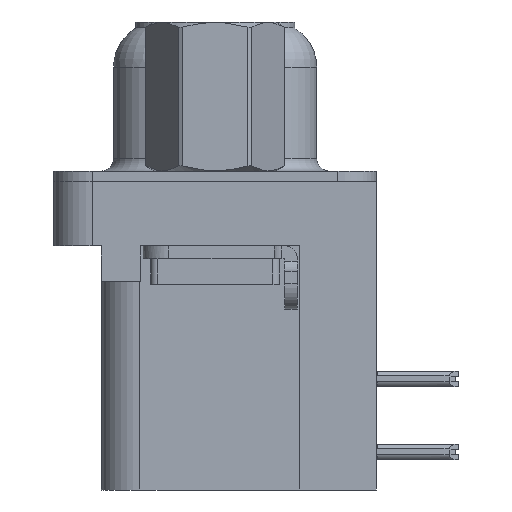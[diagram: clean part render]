
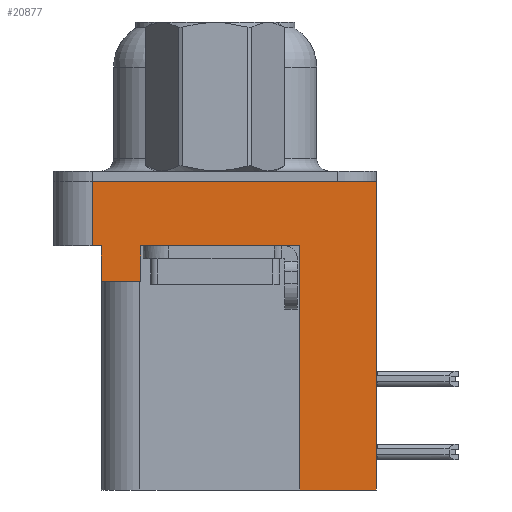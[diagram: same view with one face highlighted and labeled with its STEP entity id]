
A CAD part, left-side view. The second image highlights one B-rep face of the part: STEP entity #20877.
In plain terms, the highlighted planar face has unit normal (-1, 0, 0).
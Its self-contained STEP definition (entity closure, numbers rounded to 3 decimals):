
#188 = ORIENTED_EDGE ( 'NONE', *, *, #10107, .F. ) ;
#327 = CARTESIAN_POINT ( 'NONE',  ( -2.91, 4.425, -3.9 ) ) ;
#894 = ORIENTED_EDGE ( 'NONE', *, *, #11060, .T. ) ;
#1108 = VECTOR ( 'NONE', #5291, 1000. ) ;
#1825 = DIRECTION ( 'NONE',  ( -1., 0., 0. ) ) ;
#2499 = LINE ( 'NONE', #14747, #24921 ) ;
#2688 = VERTEX_POINT ( 'NONE', #21007 ) ;
#3097 = CARTESIAN_POINT ( 'NONE',  ( -2.91, 2.895, -3.9 ) ) ;
#3194 = CARTESIAN_POINT ( 'NONE',  ( -2.91, 4.425, -3.9 ) ) ;
#3230 = VERTEX_POINT ( 'NONE', #9483 ) ;
#3267 = EDGE_CURVE ( 'NONE', #19545, #26662, #27232, .T. ) ;
#3605 = CARTESIAN_POINT ( 'NONE',  ( -2.91, 4.775, 0. ) ) ;
#3704 = ORIENTED_EDGE ( 'NONE', *, *, #19680, .F. ) ;
#3822 = CARTESIAN_POINT ( 'NONE',  ( -2.91, 4.775, -2.5 ) ) ;
#3867 = EDGE_CURVE ( 'NONE', #12359, #3230, #27208, .T. ) ;
#4032 = LINE ( 'NONE', #10793, #15610 ) ;
#5291 = DIRECTION ( 'NONE',  ( 0., 1., 0. ) ) ;
#5613 = VECTOR ( 'NONE', #7174, 1000. ) ;
#5878 = ORIENTED_EDGE ( 'NONE', *, *, #3267, .T. ) ;
#6652 = EDGE_LOOP ( 'NONE', ( #3704, #24620, #894, #14716, #17899, #5878, #19977, #18551, #188, #24154 ) ) ;
#6826 = LINE ( 'NONE', #26333, #17709 ) ;
#6955 = LINE ( 'NONE', #3194, #1108 ) ;
#7174 = DIRECTION ( 'NONE',  ( 0., 1., 0. ) ) ;
#7348 = LINE ( 'NONE', #3822, #13152 ) ;
#9372 = LINE ( 'NONE', #327, #15237 ) ;
#9483 = CARTESIAN_POINT ( 'NONE',  ( -2.91, -3.295, -2.5 ) ) ;
#10107 = EDGE_CURVE ( 'NONE', #14349, #12359, #18548, .T. ) ;
#10502 = VECTOR ( 'NONE', #26918, 1000. ) ;
#10515 = VECTOR ( 'NONE', #14252, 1000. ) ;
#10793 = CARTESIAN_POINT ( 'NONE',  ( -2.91, -6.275, -2.5 ) ) ;
#11060 = EDGE_CURVE ( 'NONE', #25687, #16806, #6826, .T. ) ;
#11087 = DIRECTION ( 'NONE',  ( 0., -1., 0. ) ) ;
#11893 = LINE ( 'NONE', #12030, #10515 ) ;
#12030 = CARTESIAN_POINT ( 'NONE',  ( -2.91, -6.275, 0. ) ) ;
#12223 = CARTESIAN_POINT ( 'NONE',  ( -2.91, -3.295, -12. ) ) ;
#12359 = VERTEX_POINT ( 'NONE', #12223 ) ;
#12469 = EDGE_CURVE ( 'NONE', #26662, #3230, #4032, .T. ) ;
#12629 = DIRECTION ( 'NONE',  ( 0., 0., 1. ) ) ;
#13152 = VECTOR ( 'NONE', #25494, 1000. ) ;
#13293 = CARTESIAN_POINT ( 'NONE',  ( -2.91, 4.425, -2.5 ) ) ;
#13490 = EDGE_CURVE ( 'NONE', #2688, #16806, #9372, .T. ) ;
#13887 = CARTESIAN_POINT ( 'NONE',  ( -2.91, -3.295, -12. ) ) ;
#14252 = DIRECTION ( 'NONE',  ( 0., -1., 0. ) ) ;
#14349 = VERTEX_POINT ( 'NONE', #20724 ) ;
#14716 = ORIENTED_EDGE ( 'NONE', *, *, #13490, .F. ) ;
#14747 = CARTESIAN_POINT ( 'NONE',  ( -2.91, -6.275, -2.5 ) ) ;
#14824 = CARTESIAN_POINT ( 'NONE',  ( -2.91, -6.275, -2.5 ) ) ;
#15121 = VERTEX_POINT ( 'NONE', #20215 ) ;
#15237 = VECTOR ( 'NONE', #24132, 1000. ) ;
#15610 = VECTOR ( 'NONE', #26050, 1000. ) ;
#16806 = VERTEX_POINT ( 'NONE', #13293 ) ;
#17018 = DIRECTION ( 'NONE',  ( 0., 0., 1. ) ) ;
#17323 = EDGE_CURVE ( 'NONE', #14349, #15121, #2499, .T. ) ;
#17709 = VECTOR ( 'NONE', #11087, 1000. ) ;
#17899 = ORIENTED_EDGE ( 'NONE', *, *, #25410, .F. ) ;
#18149 = CARTESIAN_POINT ( 'NONE',  ( -2.91, 2.895, -3.9 ) ) ;
#18292 = DIRECTION ( 'NONE',  ( 0., 0., 1. ) ) ;
#18548 = LINE ( 'NONE', #24214, #5613 ) ;
#18551 = ORIENTED_EDGE ( 'NONE', *, *, #3867, .F. ) ;
#19545 = VERTEX_POINT ( 'NONE', #18149 ) ;
#19680 = EDGE_CURVE ( 'NONE', #25805, #15121, #11893, .T. ) ;
#19977 = ORIENTED_EDGE ( 'NONE', *, *, #12469, .T. ) ;
#20215 = CARTESIAN_POINT ( 'NONE',  ( -2.91, -6.275, 0. ) ) ;
#20724 = CARTESIAN_POINT ( 'NONE',  ( -2.91, -6.275, -12. ) ) ;
#20877 = ADVANCED_FACE ( 'NONE', ( #27194 ), #25648, .T. ) ;
#21007 = CARTESIAN_POINT ( 'NONE',  ( -2.91, 4.425, -3.9 ) ) ;
#21013 = AXIS2_PLACEMENT_3D ( 'NONE', #14824, #1825, #17018 ) ;
#21462 = VECTOR ( 'NONE', #18292, 1000. ) ;
#22141 = CARTESIAN_POINT ( 'NONE',  ( -2.91, 2.895, -2.5 ) ) ;
#23477 = EDGE_CURVE ( 'NONE', #25687, #25805, #7348, .T. ) ;
#24132 = DIRECTION ( 'NONE',  ( 0., 0., 1. ) ) ;
#24154 = ORIENTED_EDGE ( 'NONE', *, *, #17323, .T. ) ;
#24214 = CARTESIAN_POINT ( 'NONE',  ( -2.91, -3.295, -12. ) ) ;
#24538 = CARTESIAN_POINT ( 'NONE',  ( -2.91, 4.775, -2.5 ) ) ;
#24620 = ORIENTED_EDGE ( 'NONE', *, *, #23477, .F. ) ;
#24921 = VECTOR ( 'NONE', #12629, 1000. ) ;
#25410 = EDGE_CURVE ( 'NONE', #19545, #2688, #6955, .T. ) ;
#25494 = DIRECTION ( 'NONE',  ( 0., 0., 1. ) ) ;
#25648 = PLANE ( 'NONE',  #21013 ) ;
#25687 = VERTEX_POINT ( 'NONE', #24538 ) ;
#25805 = VERTEX_POINT ( 'NONE', #3605 ) ;
#26050 = DIRECTION ( 'NONE',  ( 0., -1., 0. ) ) ;
#26333 = CARTESIAN_POINT ( 'NONE',  ( -2.91, -6.275, -2.5 ) ) ;
#26662 = VERTEX_POINT ( 'NONE', #22141 ) ;
#26918 = DIRECTION ( 'NONE',  ( 0., 0., 1. ) ) ;
#27194 = FACE_OUTER_BOUND ( 'NONE', #6652, .T. ) ;
#27208 = LINE ( 'NONE', #13887, #10502 ) ;
#27232 = LINE ( 'NONE', #3097, #21462 ) ;
